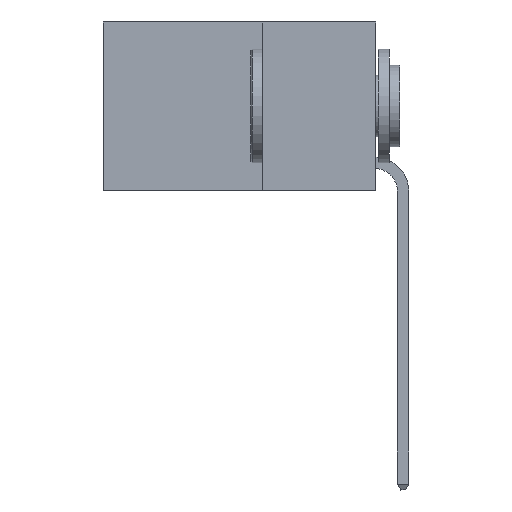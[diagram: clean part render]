
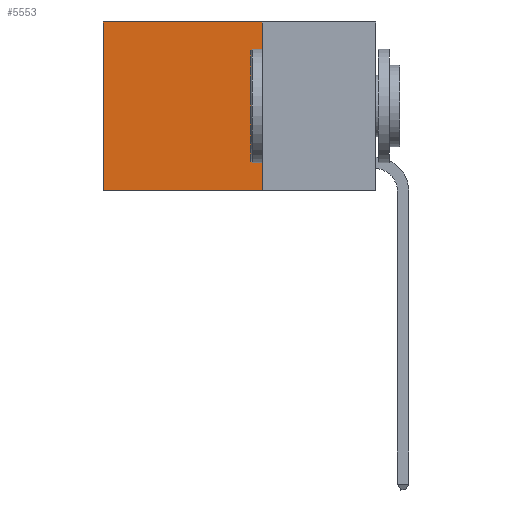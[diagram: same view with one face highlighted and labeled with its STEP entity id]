
A CAD part, left-side view. The second image highlights one B-rep face of the part: STEP entity #5553.
In plain terms, the highlighted planar face has unit normal (-1, 0, 0).
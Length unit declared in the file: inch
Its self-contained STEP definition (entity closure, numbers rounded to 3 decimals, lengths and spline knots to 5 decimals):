
#267 = CARTESIAN_POINT ( 'NONE',  ( 0.2625, 0.25, -0.37 ) ) ;
#360 = DIRECTION ( 'NONE',  ( 0., 0., -1. ) ) ;
#625 = FACE_OUTER_BOUND ( 'NONE', #3876, .T. ) ;
#1015 = DIRECTION ( 'NONE',  ( 0., 1., 0. ) ) ;
#1298 = EDGE_CURVE ( 'NONE', #3287, #7633, #7685, .T. ) ;
#1575 = ORIENTED_EDGE ( 'NONE', *, *, #3478, .T. ) ;
#1826 = LINE ( 'NONE', #3253, #5412 ) ;
#1853 = LINE ( 'NONE', #8922, #7158 ) ;
#1985 = ORIENTED_EDGE ( 'NONE', *, *, #1298, .T. ) ;
#2118 = AXIS2_PLACEMENT_3D ( 'NONE', #6342, #9190, #7781 ) ;
#3253 = CARTESIAN_POINT ( 'NONE',  ( 0.2625, 0.25, 0. ) ) ;
#3287 = VERTEX_POINT ( 'NONE', #7163 ) ;
#3442 = DIRECTION ( 'NONE',  ( 0., 1., 0. ) ) ;
#3478 = EDGE_CURVE ( 'NONE', #7633, #4873, #1853, .T. ) ;
#3493 = PLANE ( 'NONE',  #2118 ) ;
#3598 = ORIENTED_EDGE ( 'NONE', *, *, #7126, .F. ) ;
#3876 = EDGE_LOOP ( 'NONE', ( #1575, #3598, #7168, #1985 ) ) ;
#4134 = CARTESIAN_POINT ( 'NONE',  ( 0.2625, 0.25, 0. ) ) ;
#4304 = VERTEX_POINT ( 'NONE', #7498 ) ;
#4797 = VECTOR ( 'NONE', #1015, 39.37008 ) ;
#4838 = CARTESIAN_POINT ( 'NONE',  ( 0.2625, 0.6, 0. ) ) ;
#4873 = VERTEX_POINT ( 'NONE', #9059 ) ;
#5412 = VECTOR ( 'NONE', #7543, 39.37008 ) ;
#5553 = ADVANCED_FACE ( 'NONE', ( #625 ), #3493, .F. ) ;
#6342 = CARTESIAN_POINT ( 'NONE',  ( 0.2625, 0.25, 0. ) ) ;
#6740 = LINE ( 'NONE', #267, #4797 ) ;
#7126 = EDGE_CURVE ( 'NONE', #4304, #4873, #6740, .T. ) ;
#7158 = VECTOR ( 'NONE', #360, 39.37008 ) ;
#7163 = CARTESIAN_POINT ( 'NONE',  ( 0.2625, 0.25, 0. ) ) ;
#7168 = ORIENTED_EDGE ( 'NONE', *, *, #7519, .F. ) ;
#7498 = CARTESIAN_POINT ( 'NONE',  ( 0.2625, 0.25, -0.37 ) ) ;
#7519 = EDGE_CURVE ( 'NONE', #3287, #4304, #1826, .T. ) ;
#7543 = DIRECTION ( 'NONE',  ( 0., 0., -1. ) ) ;
#7633 = VERTEX_POINT ( 'NONE', #4838 ) ;
#7685 = LINE ( 'NONE', #4134, #8558 ) ;
#7781 = DIRECTION ( 'NONE',  ( 0., 0., -1. ) ) ;
#8558 = VECTOR ( 'NONE', #3442, 39.37008 ) ;
#8922 = CARTESIAN_POINT ( 'NONE',  ( 0.2625, 0.6, 0. ) ) ;
#9059 = CARTESIAN_POINT ( 'NONE',  ( 0.2625, 0.6, -0.37 ) ) ;
#9190 = DIRECTION ( 'NONE',  ( 1., 0., 0. ) ) ;
